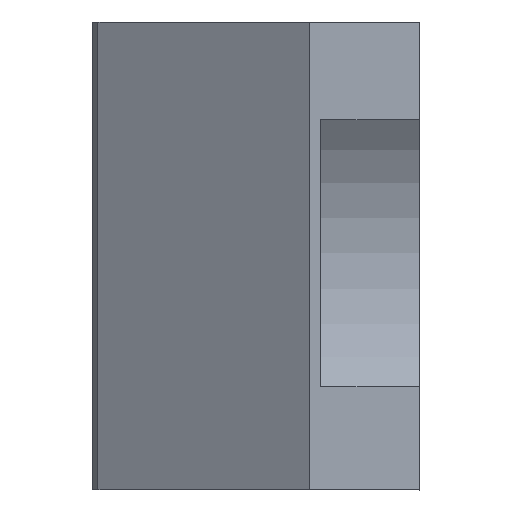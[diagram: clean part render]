
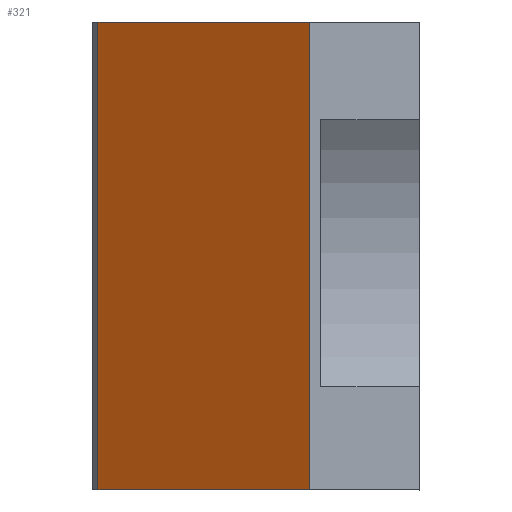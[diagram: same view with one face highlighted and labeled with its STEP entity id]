
A CAD part, top view. The second image highlights one B-rep face of the part: STEP entity #321.
In plain terms, the highlighted planar face has unit normal (-0.538, 0, 0.843).
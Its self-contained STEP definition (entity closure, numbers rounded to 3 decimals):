
#36=FACE_OUTER_BOUND('',#54,.T.);
#54=EDGE_LOOP('',(#276,#277,#278,#279));
#85=LINE('',#506,#125);
#90=LINE('',#515,#130);
#95=LINE('',#526,#135);
#97=LINE('',#529,#137);
#125=VECTOR('',#413,10.);
#130=VECTOR('',#420,10.);
#135=VECTOR('',#431,10.);
#137=VECTOR('',#435,10.);
#158=VERTEX_POINT('',#503);
#159=VERTEX_POINT('',#505);
#162=VERTEX_POINT('',#513);
#165=VERTEX_POINT('',#525);
#195=EDGE_CURVE('',#159,#158,#85,.T.);
#200=EDGE_CURVE('',#158,#162,#90,.T.);
#205=EDGE_CURVE('',#165,#159,#95,.T.);
#207=EDGE_CURVE('',#165,#162,#97,.T.);
#276=ORIENTED_EDGE('',*,*,#200,.T.);
#277=ORIENTED_EDGE('',*,*,#207,.F.);
#278=ORIENTED_EDGE('',*,*,#205,.T.);
#279=ORIENTED_EDGE('',*,*,#195,.T.);
#304=PLANE('',#355);
#321=ADVANCED_FACE('',(#36),#304,.T.);
#355=AXIS2_PLACEMENT_3D('',#528,#433,#434);
#413=DIRECTION('',(0.,1.,0.));
#420=DIRECTION('',(-0.843,0.,-0.538));
#431=DIRECTION('',(0.843,0.,0.538));
#433=DIRECTION('center_axis',(-0.538,0.,0.843));
#434=DIRECTION('ref_axis',(0.843,0.,0.538));
#435=DIRECTION('',(0.,1.,0.));
#503=CARTESIAN_POINT('',(7.82,3.5,24.089));
#505=CARTESIAN_POINT('',(7.82,-13.5,24.089));
#506=CARTESIAN_POINT('',(7.82,0.,24.089));
#513=CARTESIAN_POINT('',(0.138,3.5,19.191));
#515=CARTESIAN_POINT('',(-0.143,3.5,19.011));
#525=CARTESIAN_POINT('',(0.138,-13.5,19.191));
#526=CARTESIAN_POINT('',(4.193,-13.5,21.776));
#528=CARTESIAN_POINT('Origin',(8.374,0.,24.443));
#529=CARTESIAN_POINT('',(0.138,0.,19.191));
